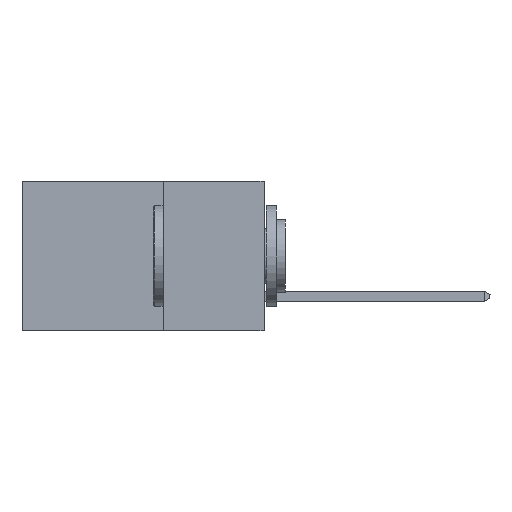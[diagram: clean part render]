
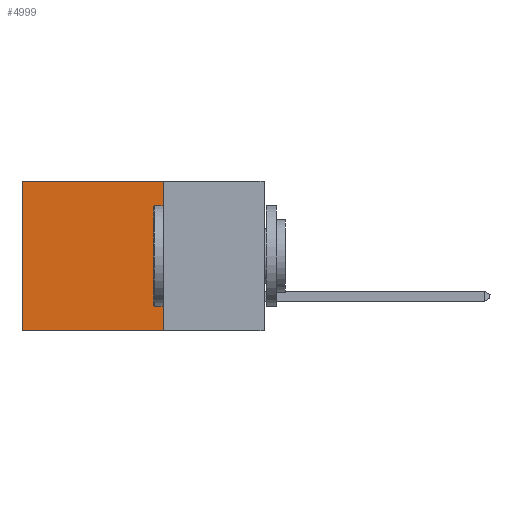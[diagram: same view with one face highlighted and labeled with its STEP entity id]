
A CAD part, left-side view. The second image highlights one B-rep face of the part: STEP entity #4999.
In plain terms, the highlighted planar face has unit normal (-1, 0, 0).
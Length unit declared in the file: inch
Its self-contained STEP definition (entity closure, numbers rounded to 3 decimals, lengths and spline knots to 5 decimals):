
#572 = DIRECTION ( 'NONE',  ( 0., 0., -1. ) ) ;
#977 = DIRECTION ( 'NONE',  ( 0., 0., -1. ) ) ;
#1322 = VECTOR ( 'NONE', #4591, 39.37008 ) ;
#1750 = DIRECTION ( 'NONE',  ( 0., 0., -1. ) ) ;
#2632 = DIRECTION ( 'NONE',  ( 0., 1., 0. ) ) ;
#2700 = CARTESIAN_POINT ( 'NONE',  ( 0.2615, 0.6, 0. ) ) ;
#3309 = ORIENTED_EDGE ( 'NONE', *, *, #10316, .T. ) ;
#3501 = DIRECTION ( 'NONE',  ( 1., 0., 0. ) ) ;
#4591 = DIRECTION ( 'NONE',  ( 0., 1., 0. ) ) ;
#4647 = ORIENTED_EDGE ( 'NONE', *, *, #10502, .T. ) ;
#4999 = ADVANCED_FACE ( 'NONE', ( #5116 ), #12564, .F. ) ;
#5116 = FACE_OUTER_BOUND ( 'NONE', #16747, .T. ) ;
#5620 = CARTESIAN_POINT ( 'NONE',  ( 0.2615, 0.6, -0.37 ) ) ;
#6785 = VECTOR ( 'NONE', #2632, 39.37008 ) ;
#6899 = CARTESIAN_POINT ( 'NONE',  ( 0.2615, 0.6, -0.37 ) ) ;
#7337 = CARTESIAN_POINT ( 'NONE',  ( 0.2615, 0.25, 0. ) ) ;
#7340 = CARTESIAN_POINT ( 'NONE',  ( 0.2615, 0.25, -0.37 ) ) ;
#7688 = ORIENTED_EDGE ( 'NONE', *, *, #12695, .F. ) ;
#8760 = VERTEX_POINT ( 'NONE', #2700 ) ;
#9678 = AXIS2_PLACEMENT_3D ( 'NONE', #11023, #3501, #572 ) ;
#10133 = EDGE_CURVE ( 'NONE', #17770, #13222, #14085, .T. ) ;
#10299 = LINE ( 'NONE', #5620, #13954 ) ;
#10316 = EDGE_CURVE ( 'NONE', #8760, #13222, #10299, .T. ) ;
#10502 = EDGE_CURVE ( 'NONE', #15855, #8760, #10704, .T. ) ;
#10704 = LINE ( 'NONE', #18555, #1322 ) ;
#11023 = CARTESIAN_POINT ( 'NONE',  ( 0.2615, 0.25, -0.37 ) ) ;
#12564 = PLANE ( 'NONE',  #9678 ) ;
#12695 = EDGE_CURVE ( 'NONE', #15855, #17770, #17228, .T. ) ;
#13222 = VERTEX_POINT ( 'NONE', #6899 ) ;
#13339 = VECTOR ( 'NONE', #1750, 39.37008 ) ;
#13954 = VECTOR ( 'NONE', #977, 39.37008 ) ;
#14085 = LINE ( 'NONE', #16578, #6785 ) ;
#15698 = CARTESIAN_POINT ( 'NONE',  ( 0.2615, 0.25, -0.37 ) ) ;
#15855 = VERTEX_POINT ( 'NONE', #7337 ) ;
#16578 = CARTESIAN_POINT ( 'NONE',  ( 0.2615, 0.25, -0.37 ) ) ;
#16747 = EDGE_LOOP ( 'NONE', ( #3309, #19084, #7688, #4647 ) ) ;
#17228 = LINE ( 'NONE', #15698, #13339 ) ;
#17770 = VERTEX_POINT ( 'NONE', #7340 ) ;
#18555 = CARTESIAN_POINT ( 'NONE',  ( 0.2615, 0.25, 0. ) ) ;
#19084 = ORIENTED_EDGE ( 'NONE', *, *, #10133, .F. ) ;
